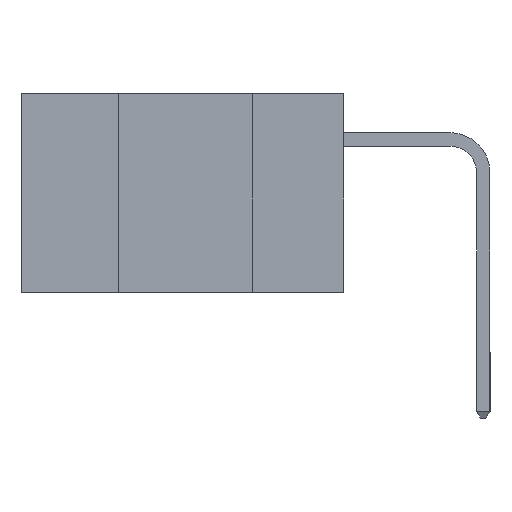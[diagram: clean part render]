
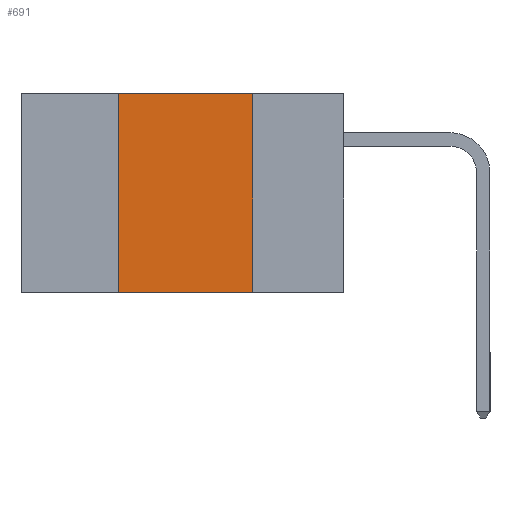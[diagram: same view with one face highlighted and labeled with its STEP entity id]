
A CAD part, left-side view. The second image highlights one B-rep face of the part: STEP entity #691.
In plain terms, the highlighted planar face has unit normal (-1, 0, 0).
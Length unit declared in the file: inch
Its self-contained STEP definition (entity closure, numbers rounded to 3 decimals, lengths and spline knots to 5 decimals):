
#420 = LINE ( 'NONE', #6396, #19088 ) ;
#691 = ADVANCED_FACE ( 'NONE', ( #15628 ), #12221, .F. ) ;
#725 = CARTESIAN_POINT ( 'NONE',  ( 0., 0.6, 0. ) ) ;
#973 = DIRECTION ( 'NONE',  ( 0., 0., -1. ) ) ;
#1834 = VECTOR ( 'NONE', #13484, 39.37008 ) ;
#4782 = CARTESIAN_POINT ( 'NONE',  ( 0., 0.42, 0. ) ) ;
#5486 = VERTEX_POINT ( 'NONE', #12487 ) ;
#6396 = CARTESIAN_POINT ( 'NONE',  ( 0., 0.17, 0. ) ) ;
#6454 = ORIENTED_EDGE ( 'NONE', *, *, #18200, .T. ) ;
#7002 = CARTESIAN_POINT ( 'NONE',  ( 0., 0.6, -0.37 ) ) ;
#7315 = EDGE_CURVE ( 'NONE', #11960, #18150, #21545, .T. ) ;
#8110 = LINE ( 'NONE', #725, #1834 ) ;
#8765 = EDGE_LOOP ( 'NONE', ( #16066, #13719, #17431, #6454 ) ) ;
#9076 = DIRECTION ( 'NONE',  ( 0., -1., 0. ) ) ;
#9156 = CARTESIAN_POINT ( 'NONE',  ( 0., 0.42, 0. ) ) ;
#9202 = VERTEX_POINT ( 'NONE', #22322 ) ;
#10504 = DIRECTION ( 'NONE',  ( 0., 0., -1. ) ) ;
#11452 = VECTOR ( 'NONE', #9076, 39.37008 ) ;
#11938 = VECTOR ( 'NONE', #18163, 39.37008 ) ;
#11960 = VERTEX_POINT ( 'NONE', #20388 ) ;
#12221 = PLANE ( 'NONE',  #14294 ) ;
#12487 = CARTESIAN_POINT ( 'NONE',  ( 0., 0.17, -0.37 ) ) ;
#13484 = DIRECTION ( 'NONE',  ( 0., -1., 0. ) ) ;
#13719 = ORIENTED_EDGE ( 'NONE', *, *, #14078, .F. ) ;
#14015 = CARTESIAN_POINT ( 'NONE',  ( 0., 0.6, 0. ) ) ;
#14078 = EDGE_CURVE ( 'NONE', #18150, #9202, #8110, .T. ) ;
#14294 = AXIS2_PLACEMENT_3D ( 'NONE', #14015, #21299, #10504 ) ;
#15628 = FACE_OUTER_BOUND ( 'NONE', #8765, .T. ) ;
#16066 = ORIENTED_EDGE ( 'NONE', *, *, #23291, .F. ) ;
#17431 = ORIENTED_EDGE ( 'NONE', *, *, #7315, .F. ) ;
#18150 = VERTEX_POINT ( 'NONE', #4782 ) ;
#18163 = DIRECTION ( 'NONE',  ( 0., 0., 1. ) ) ;
#18200 = EDGE_CURVE ( 'NONE', #11960, #5486, #19331, .T. ) ;
#19088 = VECTOR ( 'NONE', #973, 39.37008 ) ;
#19331 = LINE ( 'NONE', #7002, #11452 ) ;
#20388 = CARTESIAN_POINT ( 'NONE',  ( 0., 0.42, -0.37 ) ) ;
#21299 = DIRECTION ( 'NONE',  ( 1., 0., 0. ) ) ;
#21545 = LINE ( 'NONE', #9156, #11938 ) ;
#22322 = CARTESIAN_POINT ( 'NONE',  ( 0., 0.17, 0. ) ) ;
#23291 = EDGE_CURVE ( 'NONE', #9202, #5486, #420, .T. ) ;
